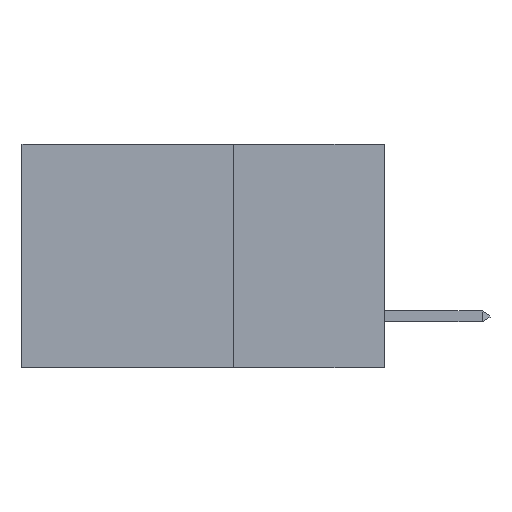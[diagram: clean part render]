
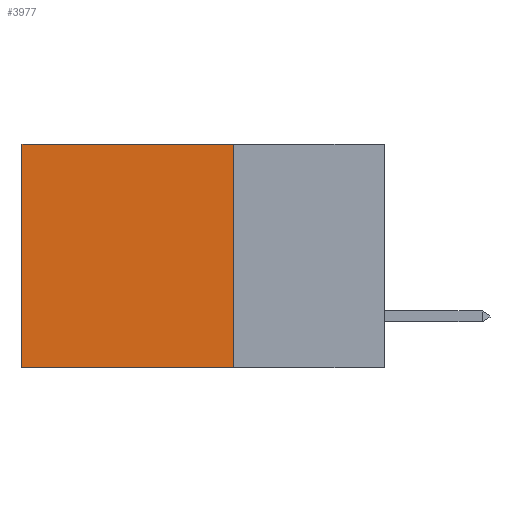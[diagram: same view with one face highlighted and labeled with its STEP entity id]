
A CAD part, left-side view. The second image highlights one B-rep face of the part: STEP entity #3977.
In plain terms, the highlighted planar face has unit normal (-1, 0, 0).
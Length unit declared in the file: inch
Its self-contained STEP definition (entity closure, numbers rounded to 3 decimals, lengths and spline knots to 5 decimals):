
#603 = EDGE_CURVE ( 'NONE', #6483, #10891, #12359, .T. ) ;
#1187 = ORIENTED_EDGE ( 'NONE', *, *, #2696, .F. ) ;
#2518 = VECTOR ( 'NONE', #12992, 39.37008 ) ;
#2696 = EDGE_CURVE ( 'NONE', #4964, #10891, #5269, .T. ) ;
#2750 = DIRECTION ( 'NONE',  ( 0., 0., -1. ) ) ;
#3376 = LINE ( 'NONE', #13651, #5611 ) ;
#3708 = VERTEX_POINT ( 'NONE', #7304 ) ;
#3977 = ADVANCED_FACE ( 'NONE', ( #9871 ), #5311, .F. ) ;
#4569 = EDGE_CURVE ( 'NONE', #3708, #4964, #3376, .T. ) ;
#4617 = CARTESIAN_POINT ( 'NONE',  ( 0.2875, 0.25, 0. ) ) ;
#4949 = ORIENTED_EDGE ( 'NONE', *, *, #4569, .F. ) ;
#4964 = VERTEX_POINT ( 'NONE', #10788 ) ;
#5269 = LINE ( 'NONE', #10559, #14378 ) ;
#5311 = PLANE ( 'NONE',  #5940 ) ;
#5536 = ORIENTED_EDGE ( 'NONE', *, *, #15584, .T. ) ;
#5598 = CARTESIAN_POINT ( 'NONE',  ( 0.2875, 0.6, 0. ) ) ;
#5611 = VECTOR ( 'NONE', #14775, 39.37008 ) ;
#5618 = CARTESIAN_POINT ( 'NONE',  ( 0.2875, 0.6, 0. ) ) ;
#5940 = AXIS2_PLACEMENT_3D ( 'NONE', #8895, #10080, #2750 ) ;
#5944 = LINE ( 'NONE', #4617, #2518 ) ;
#6483 = VERTEX_POINT ( 'NONE', #5618 ) ;
#7304 = CARTESIAN_POINT ( 'NONE',  ( 0.2875, 0.25, 0. ) ) ;
#7787 = EDGE_LOOP ( 'NONE', ( #8657, #1187, #4949, #5536 ) ) ;
#8657 = ORIENTED_EDGE ( 'NONE', *, *, #603, .T. ) ;
#8895 = CARTESIAN_POINT ( 'NONE',  ( 0.2875, 0.25, 0. ) ) ;
#9871 = FACE_OUTER_BOUND ( 'NONE', #7787, .T. ) ;
#10080 = DIRECTION ( 'NONE',  ( 1., 0., 0. ) ) ;
#10386 = DIRECTION ( 'NONE',  ( 0., 0., -1. ) ) ;
#10559 = CARTESIAN_POINT ( 'NONE',  ( 0.2875, 0.25, -0.37 ) ) ;
#10788 = CARTESIAN_POINT ( 'NONE',  ( 0.2875, 0.25, -0.37 ) ) ;
#10891 = VERTEX_POINT ( 'NONE', #13991 ) ;
#12359 = LINE ( 'NONE', #5598, #15125 ) ;
#12678 = DIRECTION ( 'NONE',  ( 0., 1., 0. ) ) ;
#12992 = DIRECTION ( 'NONE',  ( 0., 1., 0. ) ) ;
#13651 = CARTESIAN_POINT ( 'NONE',  ( 0.2875, 0.25, 0. ) ) ;
#13991 = CARTESIAN_POINT ( 'NONE',  ( 0.2875, 0.6, -0.37 ) ) ;
#14378 = VECTOR ( 'NONE', #12678, 39.37008 ) ;
#14775 = DIRECTION ( 'NONE',  ( 0., 0., -1. ) ) ;
#15125 = VECTOR ( 'NONE', #10386, 39.37008 ) ;
#15584 = EDGE_CURVE ( 'NONE', #3708, #6483, #5944, .T. ) ;
